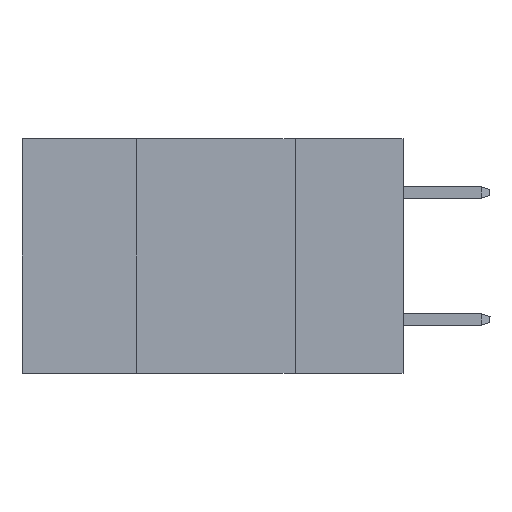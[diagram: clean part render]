
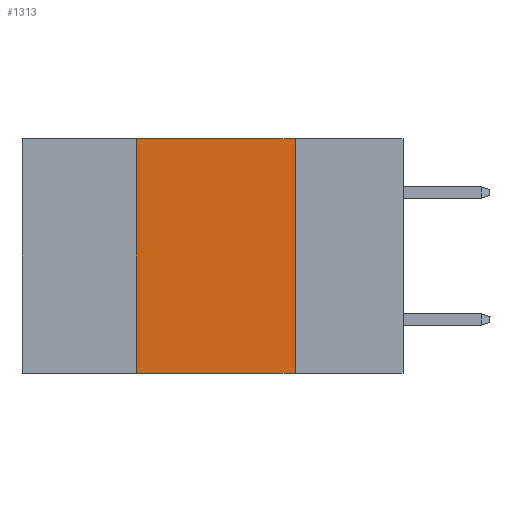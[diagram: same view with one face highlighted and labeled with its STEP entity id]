
A CAD part, left-side view. The second image highlights one B-rep face of the part: STEP entity #1313.
In plain terms, the highlighted planar face has unit normal (-1, 0, 0).
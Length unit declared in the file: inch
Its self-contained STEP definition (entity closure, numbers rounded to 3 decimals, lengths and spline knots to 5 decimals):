
#649 = CARTESIAN_POINT ( 'NONE',  ( 0., 0.17, -0.37 ) ) ;
#941 = ORIENTED_EDGE ( 'NONE', *, *, #4817, .F. ) ;
#1313 = ADVANCED_FACE ( 'NONE', ( #5547 ), #12197, .F. ) ;
#1381 = CARTESIAN_POINT ( 'NONE',  ( 0., 0.42, -0.37 ) ) ;
#1557 = DIRECTION ( 'NONE',  ( 0., 0., 1. ) ) ;
#2001 = EDGE_LOOP ( 'NONE', ( #7634, #7784, #941, #9338 ) ) ;
#2363 = EDGE_CURVE ( 'NONE', #5502, #13272, #14056, .T. ) ;
#2486 = DIRECTION ( 'NONE',  ( 0., -1., 0. ) ) ;
#2571 = DIRECTION ( 'NONE',  ( 0., 0., -1. ) ) ;
#2817 = VECTOR ( 'NONE', #2571, 39.37008 ) ;
#4562 = VERTEX_POINT ( 'NONE', #16206 ) ;
#4774 = LINE ( 'NONE', #16308, #5557 ) ;
#4817 = EDGE_CURVE ( 'NONE', #5502, #5961, #9241, .T. ) ;
#5502 = VERTEX_POINT ( 'NONE', #1381 ) ;
#5547 = FACE_OUTER_BOUND ( 'NONE', #2001, .T. ) ;
#5557 = VECTOR ( 'NONE', #16466, 39.37008 ) ;
#5961 = VERTEX_POINT ( 'NONE', #16250 ) ;
#6573 = CARTESIAN_POINT ( 'NONE',  ( 0., 0.17, 0. ) ) ;
#7634 = ORIENTED_EDGE ( 'NONE', *, *, #8703, .F. ) ;
#7784 = ORIENTED_EDGE ( 'NONE', *, *, #8319, .F. ) ;
#8319 = EDGE_CURVE ( 'NONE', #5961, #4562, #4774, .T. ) ;
#8703 = EDGE_CURVE ( 'NONE', #4562, #13272, #12875, .T. ) ;
#9241 = LINE ( 'NONE', #10877, #9298 ) ;
#9298 = VECTOR ( 'NONE', #1557, 39.37008 ) ;
#9338 = ORIENTED_EDGE ( 'NONE', *, *, #2363, .T. ) ;
#10745 = DIRECTION ( 'NONE',  ( 1., 0., 0. ) ) ;
#10834 = VECTOR ( 'NONE', #2486, 39.37008 ) ;
#10877 = CARTESIAN_POINT ( 'NONE',  ( 0., 0.42, 0. ) ) ;
#12197 = PLANE ( 'NONE',  #15725 ) ;
#12875 = LINE ( 'NONE', #6573, #2817 ) ;
#13272 = VERTEX_POINT ( 'NONE', #649 ) ;
#14056 = LINE ( 'NONE', #14136, #10834 ) ;
#14136 = CARTESIAN_POINT ( 'NONE',  ( 0., 0.6, -0.37 ) ) ;
#14855 = CARTESIAN_POINT ( 'NONE',  ( 0., 0.6, 0. ) ) ;
#14940 = DIRECTION ( 'NONE',  ( 0., 0., -1. ) ) ;
#15725 = AXIS2_PLACEMENT_3D ( 'NONE', #14855, #10745, #14940 ) ;
#16206 = CARTESIAN_POINT ( 'NONE',  ( 0., 0.17, 0. ) ) ;
#16250 = CARTESIAN_POINT ( 'NONE',  ( 0., 0.42, 0. ) ) ;
#16308 = CARTESIAN_POINT ( 'NONE',  ( 0., 0.6, 0. ) ) ;
#16466 = DIRECTION ( 'NONE',  ( 0., -1., 0. ) ) ;
